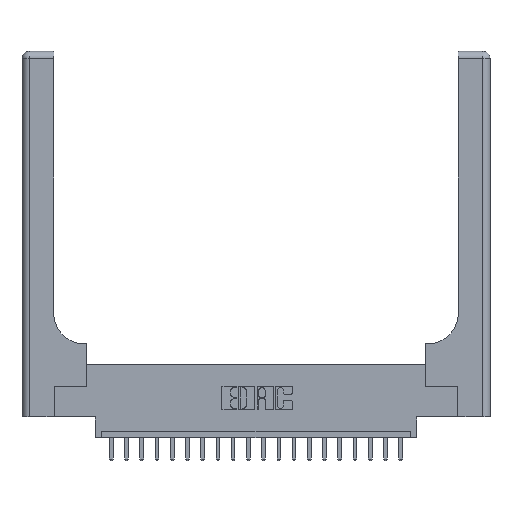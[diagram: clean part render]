
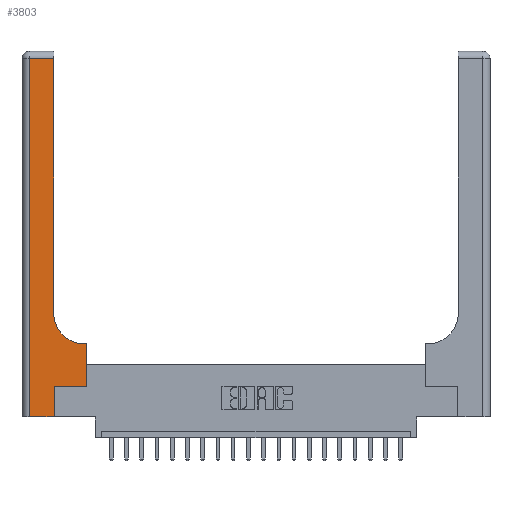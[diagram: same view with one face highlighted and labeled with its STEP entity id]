
A CAD part, top view. The second image highlights one B-rep face of the part: STEP entity #3803.
In plain terms, the highlighted planar face has unit normal (0, 0, 1).
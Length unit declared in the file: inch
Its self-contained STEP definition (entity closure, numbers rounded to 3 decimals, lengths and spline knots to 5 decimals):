
#454 = CARTESIAN_POINT ( 'NONE',  ( 0.26, 0.6, 0.37 ) ) ;
#639 = EDGE_CURVE ( 'NONE', #1912, #7340, #12128, .T. ) ;
#1577 = LINE ( 'NONE', #3182, #7154 ) ;
#1852 = VECTOR ( 'NONE', #7048, 39.37008 ) ;
#1861 = CARTESIAN_POINT ( 'NONE',  ( 0.265, 0., 0.37 ) ) ;
#1912 = VERTEX_POINT ( 'NONE', #18094 ) ;
#1991 = EDGE_CURVE ( 'NONE', #16980, #7690, #1577, .T. ) ;
#2202 = ORIENTED_EDGE ( 'NONE', *, *, #7476, .T. ) ;
#2611 = DIRECTION ( 'NONE',  ( 1., 0., 0. ) ) ;
#2832 = VECTOR ( 'NONE', #3015, 39.37008 ) ;
#3015 = DIRECTION ( 'NONE',  ( 0., -1., 0. ) ) ;
#3182 = CARTESIAN_POINT ( 'NONE',  ( 0., 2.94, 0.37 ) ) ;
#3614 = CARTESIAN_POINT ( 'NONE',  ( 0.528, 0.25, 0.37 ) ) ;
#3803 = ADVANCED_FACE ( 'NONE', ( #21250 ), #15969, .F. ) ;
#5706 = LINE ( 'NONE', #454, #15882 ) ;
#5972 = ORIENTED_EDGE ( 'NONE', *, *, #11318, .T. ) ;
#6027 = LINE ( 'NONE', #19139, #14807 ) ;
#6086 = CARTESIAN_POINT ( 'NONE',  ( 0., 3., 0.37 ) ) ;
#6167 = CARTESIAN_POINT ( 'NONE',  ( 0.51, 0.85, 0.37 ) ) ;
#6212 = VERTEX_POINT ( 'NONE', #13978 ) ;
#6456 = VECTOR ( 'NONE', #9722, 39.37008 ) ;
#7048 = DIRECTION ( 'NONE',  ( 1., 0., 0. ) ) ;
#7154 = VECTOR ( 'NONE', #9710, 39.37008 ) ;
#7340 = VERTEX_POINT ( 'NONE', #15963 ) ;
#7361 = EDGE_CURVE ( 'NONE', #6212, #7497, #10146, .T. ) ;
#7476 = EDGE_CURVE ( 'NONE', #7340, #16980, #21245, .T. ) ;
#7497 = VERTEX_POINT ( 'NONE', #13155 ) ;
#7690 = VERTEX_POINT ( 'NONE', #20482 ) ;
#7843 = CARTESIAN_POINT ( 'NONE',  ( 0.26, 2.94, 0.37 ) ) ;
#8110 = CARTESIAN_POINT ( 'NONE',  ( 0.26, 3., 0.37 ) ) ;
#8344 = AXIS2_PLACEMENT_3D ( 'NONE', #6167, #12809, #19282 ) ;
#8387 = ORIENTED_EDGE ( 'NONE', *, *, #20939, .T. ) ;
#9091 = AXIS2_PLACEMENT_3D ( 'NONE', #6086, #11245, #14246 ) ;
#9433 = LINE ( 'NONE', #15993, #2832 ) ;
#9710 = DIRECTION ( 'NONE',  ( -1., 0., 0. ) ) ;
#9722 = DIRECTION ( 'NONE',  ( 0., 1., 0. ) ) ;
#9885 = CARTESIAN_POINT ( 'NONE',  ( 0.265, 0.25, 0.37 ) ) ;
#9993 = ORIENTED_EDGE ( 'NONE', *, *, #1991, .T. ) ;
#10146 = LINE ( 'NONE', #3614, #6456 ) ;
#10910 = VECTOR ( 'NONE', #17897, 39.37008 ) ;
#11245 = DIRECTION ( 'NONE',  ( 0., 0., -1. ) ) ;
#11318 = EDGE_CURVE ( 'NONE', #14333, #18743, #15317, .T. ) ;
#11791 = VERTEX_POINT ( 'NONE', #12379 ) ;
#12128 = CIRCLE ( 'NONE', #8344, 0.25 ) ;
#12379 = CARTESIAN_POINT ( 'NONE',  ( 0.06, 0., 0.37 ) ) ;
#12809 = DIRECTION ( 'NONE',  ( 0., 0., -1. ) ) ;
#13155 = CARTESIAN_POINT ( 'NONE',  ( 0.528, 0.6, 0.37 ) ) ;
#13699 = LINE ( 'NONE', #15421, #1852 ) ;
#13978 = CARTESIAN_POINT ( 'NONE',  ( 0.528, 0.25, 0.37 ) ) ;
#14246 = DIRECTION ( 'NONE',  ( -1., 0., 0. ) ) ;
#14333 = VERTEX_POINT ( 'NONE', #1861 ) ;
#14807 = VECTOR ( 'NONE', #2611, 39.37008 ) ;
#15317 = LINE ( 'NONE', #20498, #16105 ) ;
#15408 = ORIENTED_EDGE ( 'NONE', *, *, #639, .T. ) ;
#15421 = CARTESIAN_POINT ( 'NONE',  ( 0., 0., 0.37 ) ) ;
#15586 = EDGE_CURVE ( 'NONE', #7497, #1912, #5706, .T. ) ;
#15633 = EDGE_CURVE ( 'NONE', #18743, #6212, #6027, .T. ) ;
#15882 = VECTOR ( 'NONE', #20013, 39.37008 ) ;
#15963 = CARTESIAN_POINT ( 'NONE',  ( 0.26, 0.85, 0.37 ) ) ;
#15969 = PLANE ( 'NONE',  #9091 ) ;
#15993 = CARTESIAN_POINT ( 'NONE',  ( 0.06, 3., 0.37 ) ) ;
#16105 = VECTOR ( 'NONE', #20166, 39.37008 ) ;
#16980 = VERTEX_POINT ( 'NONE', #7843 ) ;
#17304 = ORIENTED_EDGE ( 'NONE', *, *, #17734, .T. ) ;
#17734 = EDGE_CURVE ( 'NONE', #7690, #11791, #9433, .T. ) ;
#17897 = DIRECTION ( 'NONE',  ( 0., 1., 0. ) ) ;
#18094 = CARTESIAN_POINT ( 'NONE',  ( 0.51, 0.6, 0.37 ) ) ;
#18181 = EDGE_LOOP ( 'NONE', ( #2202, #9993, #17304, #8387, #5972, #20819, #18869, #20794, #15408 ) ) ;
#18743 = VERTEX_POINT ( 'NONE', #9885 ) ;
#18869 = ORIENTED_EDGE ( 'NONE', *, *, #7361, .T. ) ;
#19139 = CARTESIAN_POINT ( 'NONE',  ( 0.265, 0.25, 0.37 ) ) ;
#19282 = DIRECTION ( 'NONE',  ( 1., 0., 0. ) ) ;
#20013 = DIRECTION ( 'NONE',  ( -1., 0., 0. ) ) ;
#20166 = DIRECTION ( 'NONE',  ( 0., 1., 0. ) ) ;
#20482 = CARTESIAN_POINT ( 'NONE',  ( 0.06, 2.94, 0.37 ) ) ;
#20498 = CARTESIAN_POINT ( 'NONE',  ( 0.265, 0., 0.37 ) ) ;
#20794 = ORIENTED_EDGE ( 'NONE', *, *, #15586, .T. ) ;
#20819 = ORIENTED_EDGE ( 'NONE', *, *, #15633, .T. ) ;
#20939 = EDGE_CURVE ( 'NONE', #11791, #14333, #13699, .T. ) ;
#21245 = LINE ( 'NONE', #8110, #10910 ) ;
#21250 = FACE_OUTER_BOUND ( 'NONE', #18181, .T. ) ;
